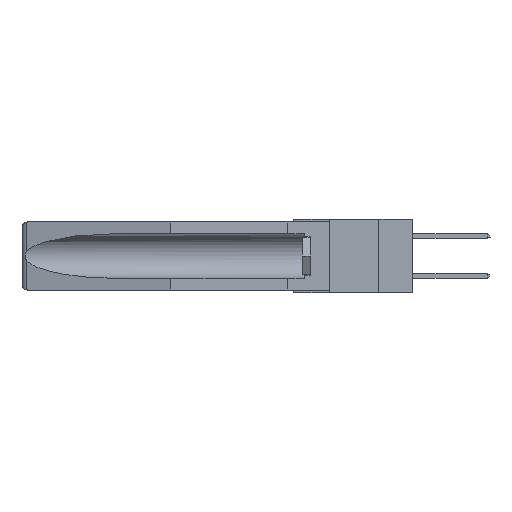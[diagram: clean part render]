
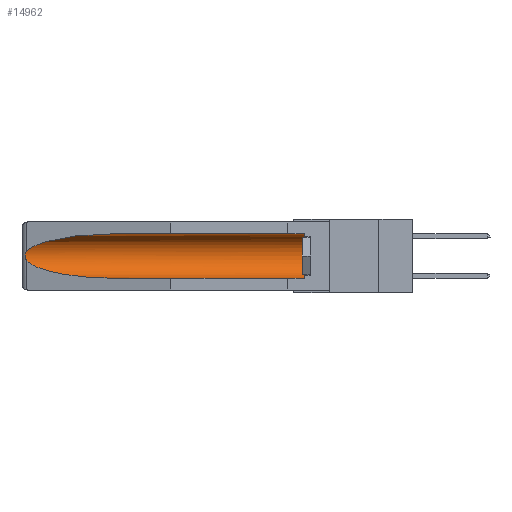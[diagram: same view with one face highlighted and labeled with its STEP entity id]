
A CAD part, left-side view. The second image highlights one B-rep face of the part: STEP entity #14962.
In plain terms, the highlighted cylindrical face has radius 2.857 mm (diameter 5.715 mm), a partial arc.
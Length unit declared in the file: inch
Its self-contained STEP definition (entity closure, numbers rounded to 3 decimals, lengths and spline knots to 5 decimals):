
#1065 = CARTESIAN_POINT ( 'NONE',  ( 0.155, 1.07973, -0.059 ) ) ;
#2602 = VECTOR ( 'NONE', #32575, 39.37008 ) ;
#3264 = DIRECTION ( 'NONE',  ( 0., -1., 0. ) ) ;
#3553 = CARTESIAN_POINT ( 'NONE',  ( 0.26537, 1.52718, -0.14972 ) ) ;
#3708 = CARTESIAN_POINT ( 'NONE',  ( 0.26537, 1.52718, -0.14972 ) ) ;
#3733 = CARTESIAN_POINT ( 'NONE',  ( 0.26537, 1.52718, -0.19328 ) ) ;
#4480 = ORIENTED_EDGE ( 'NONE', *, *, #14135, .F. ) ;
#4543 = VERTEX_POINT ( 'NONE', #3733 ) ;
#5870 = FACE_OUTER_BOUND ( 'NONE', #32461, .T. ) ;
#6221 = CARTESIAN_POINT ( 'NONE',  ( 0.26597, 1.52961, -0.15275 ) ) ;
#6400 = DIRECTION ( 'NONE',  ( 0., 1., 0. ) ) ;
#6682 =( BOUNDED_CURVE ( )  B_SPLINE_CURVE ( 3, ( #1065, #14509, #16859, #3708 ),
 .UNSPECIFIED., .F., .T. ) 
 B_SPLINE_CURVE_WITH_KNOTS ( ( 4, 4 ),
 ( 4.71239, 6.08839 ),
 .UNSPECIFIED. ) 
 CURVE ( )  GEOMETRIC_REPRESENTATION_ITEM ( )  RATIONAL_B_SPLINE_CURVE ( ( 1., 0.848, 0.848, 1. ) ) 
 REPRESENTATION_ITEM ( '' )  );
#7104 =( BOUNDED_CURVE ( )  B_SPLINE_CURVE ( 3, ( #23728, #15714, #31883, #34439 ),
 .UNSPECIFIED., .F., .F. ) 
 B_SPLINE_CURVE_WITH_KNOTS ( ( 4, 4 ),
 ( 0.1948, 1.5708 ),
 .UNSPECIFIED. ) 
 CURVE ( )  GEOMETRIC_REPRESENTATION_ITEM ( )  RATIONAL_B_SPLINE_CURVE ( ( 1., 0.848, 0.848, 1. ) ) 
 REPRESENTATION_ITEM ( '' )  );
#7359 = ORIENTED_EDGE ( 'NONE', *, *, #17301, .T. ) ;
#7397 = ORIENTED_EDGE ( 'NONE', *, *, #12564, .T. ) ;
#7627 = ORIENTED_EDGE ( 'NONE', *, *, #19344, .T. ) ;
#8014 = CARTESIAN_POINT ( 'NONE',  ( 0.155, 1.07973, -0.059 ) ) ;
#8240 = CARTESIAN_POINT ( 'NONE',  ( 0.26537, 1.52718, -0.14972 ) ) ;
#8448 = LINE ( 'NONE', #13906, #17133 ) ;
#9374 = CARTESIAN_POINT ( 'NONE',  ( 0.2673, 1.53269, -0.17917 ) ) ;
#9621 = CYLINDRICAL_SURFACE ( 'NONE', #31720, 0.1125 ) ;
#10566 = DIRECTION ( 'NONE',  ( 0., 0., 1. ) ) ;
#10990 = CARTESIAN_POINT ( 'NONE',  ( 0.155, -0.30754, -0.059 ) ) ;
#11697 = ORIENTED_EDGE ( 'NONE', *, *, #12769, .T. ) ;
#12564 = EDGE_CURVE ( 'NONE', #4543, #30718, #7104, .T. ) ;
#12769 = EDGE_CURVE ( 'NONE', #27435, #4543, #14745, .T. ) ;
#12896 = VERTEX_POINT ( 'NONE', #26748 ) ;
#12966 = CARTESIAN_POINT ( 'NONE',  ( 0.155, 1.07973, -0.284 ) ) ;
#13906 = CARTESIAN_POINT ( 'NONE',  ( 0.155, -0.30754, -0.284 ) ) ;
#14135 = EDGE_CURVE ( 'NONE', #16269, #30718, #8448, .T. ) ;
#14509 = CARTESIAN_POINT ( 'NONE',  ( 0.21114, 1.30732, -0.059 ) ) ;
#14745 = B_SPLINE_CURVE_WITH_KNOTS ( 'NONE', 3,
 ( #8240, #6221, #22616, #22744, #33458, #25351, #9374, #30688, #25464, #30919 ),
 .UNSPECIFIED., .F., .F.,
 ( 4, 2, 2, 2, 4 ),
 ( 0., 0.00029, 0.00058, 0.00087, 0.00117 ),
 .UNSPECIFIED. ) ;
#14843 = AXIS2_PLACEMENT_3D ( 'NONE', #16543, #3264, #27993 ) ;
#14962 = ADVANCED_FACE ( 'NONE', ( #5870 ), #9621, .F. ) ;
#15714 = CARTESIAN_POINT ( 'NONE',  ( 0.25451, 1.48313, -0.24835 ) ) ;
#16269 = VERTEX_POINT ( 'NONE', #29568 ) ;
#16543 = CARTESIAN_POINT ( 'NONE',  ( 0.155, 0.126, -0.1715 ) ) ;
#16859 = CARTESIAN_POINT ( 'NONE',  ( 0.25451, 1.48313, -0.09465 ) ) ;
#17133 = VECTOR ( 'NONE', #6400, 39.37008 ) ;
#17301 = EDGE_CURVE ( 'NONE', #23954, #27435, #6682, .T. ) ;
#18340 = DIRECTION ( 'NONE',  ( 0., 1., 0. ) ) ;
#18831 = LINE ( 'NONE', #10990, #2602 ) ;
#19344 = EDGE_CURVE ( 'NONE', #12896, #23954, #18831, .T. ) ;
#21056 = CIRCLE ( 'NONE', #14843, 0.1125 ) ;
#21127 = ORIENTED_EDGE ( 'NONE', *, *, #24369, .T. ) ;
#22616 = CARTESIAN_POINT ( 'NONE',  ( 0.26654, 1.53092, -0.15636 ) ) ;
#22744 = CARTESIAN_POINT ( 'NONE',  ( 0.2673, 1.5327, -0.16383 ) ) ;
#23728 = CARTESIAN_POINT ( 'NONE',  ( 0.26537, 1.52718, -0.19328 ) ) ;
#23954 = VERTEX_POINT ( 'NONE', #8014 ) ;
#24369 = EDGE_CURVE ( 'NONE', #16269, #12896, #21056, .T. ) ;
#25351 = CARTESIAN_POINT ( 'NONE',  ( 0.2675, 1.53308, -0.17534 ) ) ;
#25464 = CARTESIAN_POINT ( 'NONE',  ( 0.26597, 1.5296, -0.19026 ) ) ;
#26690 = CARTESIAN_POINT ( 'NONE',  ( 0.155, -0.30754, -0.1715 ) ) ;
#26748 = CARTESIAN_POINT ( 'NONE',  ( 0.155, 0.126, -0.059 ) ) ;
#27435 = VERTEX_POINT ( 'NONE', #3553 ) ;
#27993 = DIRECTION ( 'NONE',  ( 0., 0., 1. ) ) ;
#29568 = CARTESIAN_POINT ( 'NONE',  ( 0.155, 0.126, -0.284 ) ) ;
#30688 = CARTESIAN_POINT ( 'NONE',  ( 0.26655, 1.53094, -0.18657 ) ) ;
#30718 = VERTEX_POINT ( 'NONE', #12966 ) ;
#30919 = CARTESIAN_POINT ( 'NONE',  ( 0.26537, 1.52718, -0.19328 ) ) ;
#31720 = AXIS2_PLACEMENT_3D ( 'NONE', #26690, #18340, #10566 ) ;
#31883 = CARTESIAN_POINT ( 'NONE',  ( 0.21114, 1.30732, -0.284 ) ) ;
#32461 = EDGE_LOOP ( 'NONE', ( #7359, #11697, #7397, #4480, #21127, #7627 ) ) ;
#32575 = DIRECTION ( 'NONE',  ( 0., 1., 0. ) ) ;
#33458 = CARTESIAN_POINT ( 'NONE',  ( 0.2675, 1.53308, -0.16763 ) ) ;
#34439 = CARTESIAN_POINT ( 'NONE',  ( 0.155, 1.07973, -0.284 ) ) ;
